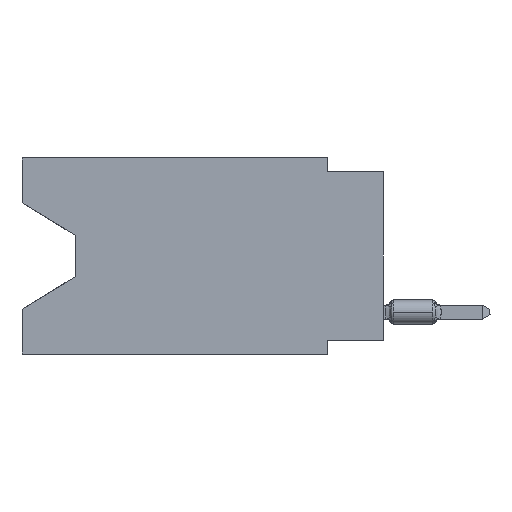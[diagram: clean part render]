
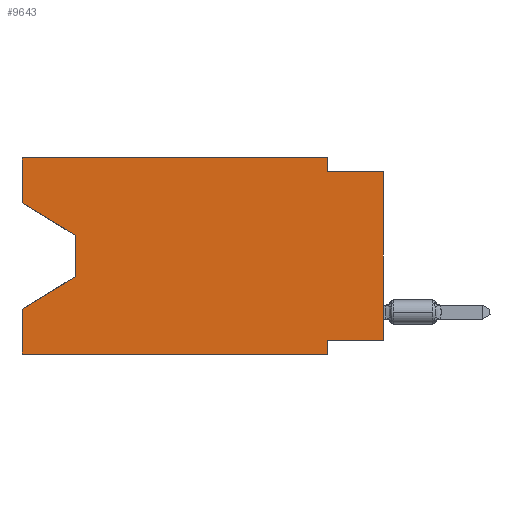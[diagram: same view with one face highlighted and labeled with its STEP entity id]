
A CAD part, left-side view. The second image highlights one B-rep face of the part: STEP entity #9643.
In plain terms, the highlighted planar face has unit normal (-1, 0, 0).
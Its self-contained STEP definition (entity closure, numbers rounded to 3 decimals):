
#538 = EDGE_CURVE ( 'NONE', #76533, #27652, #73380, .T. ) ;
#3007 = CARTESIAN_POINT ( 'NONE',  ( 0., 2.54, -8.255 ) ) ;
#3785 = VERTEX_POINT ( 'NONE', #3007 ) ;
#4256 = EDGE_CURVE ( 'NONE', #65775, #76533, #64330, .T. ) ;
#4520 = CARTESIAN_POINT ( 'NONE',  ( 0., 0., -8.255 ) ) ;
#4792 = LINE ( 'NONE', #70554, #59682 ) ;
#4938 = VECTOR ( 'NONE', #75272, 1000. ) ;
#5045 = EDGE_CURVE ( 'NONE', #19637, #20346, #4792, .T. ) ;
#5568 = LINE ( 'NONE', #22153, #79129 ) ;
#6646 = VECTOR ( 'NONE', #38701, 1000. ) ;
#7376 = DIRECTION ( 'NONE',  ( 0., -1., 0. ) ) ;
#9643 = ADVANCED_FACE ( 'NONE', ( #102101 ), #28396, .F. ) ;
#11001 = CARTESIAN_POINT ( 'NONE',  ( 0., 16.383, 0. ) ) ;
#11474 = VERTEX_POINT ( 'NONE', #69307 ) ;
#11526 = DIRECTION ( 'NONE',  ( 0., 0., 1. ) ) ;
#11982 = ORIENTED_EDGE ( 'NONE', *, *, #56947, .T. ) ;
#14307 = CARTESIAN_POINT ( 'NONE',  ( 0., 2.54, -0.635 ) ) ;
#14667 = DIRECTION ( 'NONE',  ( 0., -0.855, -0.519 ) ) ;
#14887 = CARTESIAN_POINT ( 'NONE',  ( 0., 16.383, -8.89 ) ) ;
#16767 = DIRECTION ( 'NONE',  ( 0., 0., -1. ) ) ;
#18386 = DIRECTION ( 'NONE',  ( 1., 0., 0. ) ) ;
#18615 = LINE ( 'NONE', #51759, #38535 ) ;
#19637 = VERTEX_POINT ( 'NONE', #99746 ) ;
#20346 = VERTEX_POINT ( 'NONE', #72920 ) ;
#21052 = EDGE_LOOP ( 'NONE', ( #11982, #72995, #74946, #62069, #53165, #54992, #104953, #103474, #65650, #68001, #40541, #69463 ) ) ;
#22153 = CARTESIAN_POINT ( 'NONE',  ( 0., 16.383, -2.038 ) ) ;
#23175 = CARTESIAN_POINT ( 'NONE',  ( 0., 16.383, 0. ) ) ;
#24738 = CARTESIAN_POINT ( 'NONE',  ( 0., 2.54, 0. ) ) ;
#27652 = VERTEX_POINT ( 'NONE', #14307 ) ;
#28396 = PLANE ( 'NONE',  #74311 ) ;
#28920 = CARTESIAN_POINT ( 'NONE',  ( 0., 16.383, 0. ) ) ;
#29479 = EDGE_CURVE ( 'NONE', #3785, #11474, #89995, .T. ) ;
#29714 = CARTESIAN_POINT ( 'NONE',  ( 0., 0., 0. ) ) ;
#30764 = DIRECTION ( 'NONE',  ( 0., 0., 1. ) ) ;
#33721 = VECTOR ( 'NONE', #55046, 1000. ) ;
#33899 = EDGE_CURVE ( 'NONE', #36760, #3785, #35098, .T. ) ;
#35098 = LINE ( 'NONE', #60716, #58775 ) ;
#35198 = LINE ( 'NONE', #84337, #4938 ) ;
#36173 = EDGE_CURVE ( 'NONE', #50414, #65775, #35198, .T. ) ;
#36671 = VECTOR ( 'NONE', #7376, 1000. ) ;
#36760 = VERTEX_POINT ( 'NONE', #4520 ) ;
#38535 = VECTOR ( 'NONE', #66208, 1000. ) ;
#38701 = DIRECTION ( 'NONE',  ( 0., -1., 0. ) ) ;
#40541 = ORIENTED_EDGE ( 'NONE', *, *, #4256, .F. ) ;
#41049 = VERTEX_POINT ( 'NONE', #66058 ) ;
#43634 = LINE ( 'NONE', #11001, #65699 ) ;
#48878 = CARTESIAN_POINT ( 'NONE',  ( 0., 16.383, -8.89 ) ) ;
#50414 = VERTEX_POINT ( 'NONE', #104293 ) ;
#51759 = CARTESIAN_POINT ( 'NONE',  ( 0., 0., -0.635 ) ) ;
#53165 = ORIENTED_EDGE ( 'NONE', *, *, #97016, .T. ) ;
#53763 = CARTESIAN_POINT ( 'NONE',  ( 0., 13.97, -5.385 ) ) ;
#54690 = EDGE_CURVE ( 'NONE', #20346, #67545, #92775, .T. ) ;
#54992 = ORIENTED_EDGE ( 'NONE', *, *, #29479, .F. ) ;
#55046 = DIRECTION ( 'NONE',  ( 0., 0., -1. ) ) ;
#55841 = CARTESIAN_POINT ( 'NONE',  ( 0., 2.54, -8.89 ) ) ;
#56752 = VECTOR ( 'NONE', #30764, 1000. ) ;
#56947 = EDGE_CURVE ( 'NONE', #50414, #19637, #5568, .T. ) ;
#58775 = VECTOR ( 'NONE', #102352, 1000. ) ;
#59682 = VECTOR ( 'NONE', #95134, 1000. ) ;
#60716 = CARTESIAN_POINT ( 'NONE',  ( 0., 0., -8.255 ) ) ;
#60813 = EDGE_CURVE ( 'NONE', #27652, #41049, #18615, .T. ) ;
#62069 = ORIENTED_EDGE ( 'NONE', *, *, #88771, .F. ) ;
#64330 = LINE ( 'NONE', #23175, #6646 ) ;
#65650 = ORIENTED_EDGE ( 'NONE', *, *, #60813, .F. ) ;
#65699 = VECTOR ( 'NONE', #11526, 1000. ) ;
#65775 = VERTEX_POINT ( 'NONE', #105749 ) ;
#66058 = CARTESIAN_POINT ( 'NONE',  ( 0., 0., -0.635 ) ) ;
#66208 = DIRECTION ( 'NONE',  ( 0., -1., 0. ) ) ;
#66662 = CARTESIAN_POINT ( 'NONE',  ( 0., 2.54, 0. ) ) ;
#67545 = VERTEX_POINT ( 'NONE', #101671 ) ;
#68001 = ORIENTED_EDGE ( 'NONE', *, *, #538, .F. ) ;
#69307 = CARTESIAN_POINT ( 'NONE',  ( 0., 2.54, -8.89 ) ) ;
#69463 = ORIENTED_EDGE ( 'NONE', *, *, #36173, .F. ) ;
#70085 = EDGE_CURVE ( 'NONE', #36760, #41049, #87413, .T. ) ;
#70554 = CARTESIAN_POINT ( 'NONE',  ( 0., 13.97, -3.505 ) ) ;
#72920 = CARTESIAN_POINT ( 'NONE',  ( 0., 13.97, -5.385 ) ) ;
#72995 = ORIENTED_EDGE ( 'NONE', *, *, #5045, .T. ) ;
#73380 = LINE ( 'NONE', #24738, #33721 ) ;
#74311 = AXIS2_PLACEMENT_3D ( 'NONE', #28920, #18386, #83086 ) ;
#74946 = ORIENTED_EDGE ( 'NONE', *, *, #54690, .T. ) ;
#75272 = DIRECTION ( 'NONE',  ( 0., 0., 1. ) ) ;
#76533 = VERTEX_POINT ( 'NONE', #66662 ) ;
#77054 = VECTOR ( 'NONE', #84239, 1000. ) ;
#79129 = VECTOR ( 'NONE', #14667, 1000. ) ;
#81564 = VERTEX_POINT ( 'NONE', #48878 ) ;
#83086 = DIRECTION ( 'NONE',  ( 0., 0., -1. ) ) ;
#84239 = DIRECTION ( 'NONE',  ( 0., 0.855, -0.519 ) ) ;
#84337 = CARTESIAN_POINT ( 'NONE',  ( 0., 16.383, 0. ) ) ;
#87413 = LINE ( 'NONE', #29714, #56752 ) ;
#88130 = LINE ( 'NONE', #14887, #36671 ) ;
#88771 = EDGE_CURVE ( 'NONE', #81564, #67545, #43634, .T. ) ;
#89995 = LINE ( 'NONE', #55841, #95499 ) ;
#92775 = LINE ( 'NONE', #53763, #77054 ) ;
#95134 = DIRECTION ( 'NONE',  ( 0., 0., -1. ) ) ;
#95499 = VECTOR ( 'NONE', #16767, 1000. ) ;
#97016 = EDGE_CURVE ( 'NONE', #81564, #11474, #88130, .T. ) ;
#99746 = CARTESIAN_POINT ( 'NONE',  ( 0., 13.97, -3.505 ) ) ;
#101671 = CARTESIAN_POINT ( 'NONE',  ( 0., 16.383, -6.852 ) ) ;
#102101 = FACE_OUTER_BOUND ( 'NONE', #21052, .T. ) ;
#102352 = DIRECTION ( 'NONE',  ( 0., 1., 0. ) ) ;
#103474 = ORIENTED_EDGE ( 'NONE', *, *, #70085, .T. ) ;
#104293 = CARTESIAN_POINT ( 'NONE',  ( 0., 16.383, -2.038 ) ) ;
#104953 = ORIENTED_EDGE ( 'NONE', *, *, #33899, .F. ) ;
#105749 = CARTESIAN_POINT ( 'NONE',  ( 0., 16.383, 0. ) ) ;
